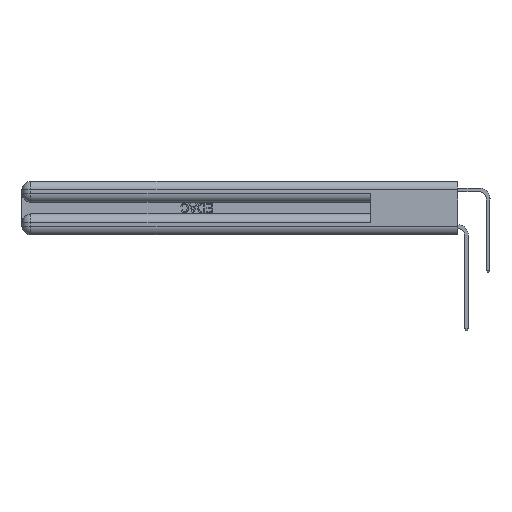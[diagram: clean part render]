
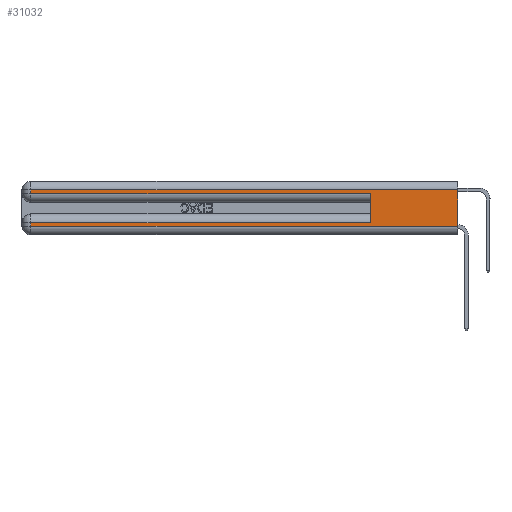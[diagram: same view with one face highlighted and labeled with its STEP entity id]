
A CAD part, left-side view. The second image highlights one B-rep face of the part: STEP entity #31032.
In plain terms, the highlighted planar face has unit normal (-1, 0, 0).
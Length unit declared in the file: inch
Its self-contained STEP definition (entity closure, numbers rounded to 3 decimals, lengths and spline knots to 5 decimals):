
#1410 = CARTESIAN_POINT ( 'NONE',  ( 0., 0.6, 0.285 ) ) ;
#1420 = ORIENTED_EDGE ( 'NONE', *, *, #5340, .F. ) ;
#1975 = LINE ( 'NONE', #37685, #36923 ) ;
#2135 = EDGE_CURVE ( 'NONE', #2789, #23034, #30403, .T. ) ;
#2245 = CARTESIAN_POINT ( 'NONE',  ( 0., 0., 0.285 ) ) ;
#2318 = EDGE_CURVE ( 'NONE', #9888, #27276, #2794, .T. ) ;
#2332 = VERTEX_POINT ( 'NONE', #26766 ) ;
#2610 = LINE ( 'NONE', #7416, #29763 ) ;
#2789 = VERTEX_POINT ( 'NONE', #29094 ) ;
#2794 = LINE ( 'NONE', #20740, #29479 ) ;
#3130 = CARTESIAN_POINT ( 'NONE',  ( 0., 2.94, 0.37 ) ) ;
#3451 = DIRECTION ( 'NONE',  ( 0., -1., 0. ) ) ;
#5340 = EDGE_CURVE ( 'NONE', #2789, #8459, #2610, .T. ) ;
#5794 = ORIENTED_EDGE ( 'NONE', *, *, #6654, .T. ) ;
#6057 = CARTESIAN_POINT ( 'NONE',  ( 0., 0., 0.06 ) ) ;
#6654 = EDGE_CURVE ( 'NONE', #16274, #27276, #7109, .T. ) ;
#6987 = CARTESIAN_POINT ( 'NONE',  ( 0., 0., 0.37 ) ) ;
#6991 = DIRECTION ( 'NONE',  ( 0., 1., 0. ) ) ;
#7109 = LINE ( 'NONE', #2245, #21837 ) ;
#7416 = CARTESIAN_POINT ( 'NONE',  ( 0., 0., 0.37 ) ) ;
#7418 = CARTESIAN_POINT ( 'NONE',  ( 0., 0.6, 0.085 ) ) ;
#8459 = VERTEX_POINT ( 'NONE', #6057 ) ;
#9888 = VERTEX_POINT ( 'NONE', #7418 ) ;
#10549 = VECTOR ( 'NONE', #19092, 39.37008 ) ;
#12088 = VECTOR ( 'NONE', #16734, 39.37008 ) ;
#12294 = DIRECTION ( 'NONE',  ( 0., 0., -1. ) ) ;
#13948 = LINE ( 'NONE', #14042, #12088 ) ;
#14042 = CARTESIAN_POINT ( 'NONE',  ( 0., 2.94, 0.37 ) ) ;
#15916 = DIRECTION ( 'NONE',  ( 0., 0., -1. ) ) ;
#15977 = EDGE_CURVE ( 'NONE', #9888, #2332, #22046, .T. ) ;
#16274 = VERTEX_POINT ( 'NONE', #29886 ) ;
#16606 = AXIS2_PLACEMENT_3D ( 'NONE', #6987, #29884, #12294 ) ;
#16734 = DIRECTION ( 'NONE',  ( 0., 0., -1. ) ) ;
#18335 = ORIENTED_EDGE ( 'NONE', *, *, #2135, .T. ) ;
#18462 = VECTOR ( 'NONE', #6991, 39.37008 ) ;
#19092 = DIRECTION ( 'NONE',  ( 0., 1., 0. ) ) ;
#20740 = CARTESIAN_POINT ( 'NONE',  ( 0., 0.6, 0.145 ) ) ;
#21837 = VECTOR ( 'NONE', #22852, 39.37008 ) ;
#22046 = LINE ( 'NONE', #36544, #10549 ) ;
#22135 = ORIENTED_EDGE ( 'NONE', *, *, #2318, .F. ) ;
#22368 = EDGE_CURVE ( 'NONE', #31572, #8459, #1975, .T. ) ;
#22852 = DIRECTION ( 'NONE',  ( 0., -1., 0. ) ) ;
#23034 = VERTEX_POINT ( 'NONE', #25589 ) ;
#23231 = DIRECTION ( 'NONE',  ( 0., 0., -1. ) ) ;
#23491 = CARTESIAN_POINT ( 'NONE',  ( 0., 0., 0.31 ) ) ;
#24449 = LINE ( 'NONE', #3130, #35050 ) ;
#24600 = PLANE ( 'NONE',  #16606 ) ;
#25589 = CARTESIAN_POINT ( 'NONE',  ( 0., 2.94, 0.31 ) ) ;
#26766 = CARTESIAN_POINT ( 'NONE',  ( 0., 2.94, 0.085 ) ) ;
#27276 = VERTEX_POINT ( 'NONE', #1410 ) ;
#29094 = CARTESIAN_POINT ( 'NONE',  ( 0., 0., 0.31 ) ) ;
#29373 = DIRECTION ( 'NONE',  ( 0., 0., 1. ) ) ;
#29479 = VECTOR ( 'NONE', #29373, 39.37008 ) ;
#29763 = VECTOR ( 'NONE', #15916, 39.37008 ) ;
#29884 = DIRECTION ( 'NONE',  ( 1., 0., 0. ) ) ;
#29886 = CARTESIAN_POINT ( 'NONE',  ( 0., 2.94, 0.285 ) ) ;
#30403 = LINE ( 'NONE', #23491, #18462 ) ;
#31032 = ADVANCED_FACE ( 'NONE', ( #32765 ), #24600, .F. ) ;
#31572 = VERTEX_POINT ( 'NONE', #33398 ) ;
#31779 = ORIENTED_EDGE ( 'NONE', *, *, #15977, .T. ) ;
#32765 = FACE_OUTER_BOUND ( 'NONE', #33131, .T. ) ;
#33131 = EDGE_LOOP ( 'NONE', ( #1420, #18335, #33409, #5794, #22135, #31779, #35691, #34311 ) ) ;
#33398 = CARTESIAN_POINT ( 'NONE',  ( 0., 2.94, 0.06 ) ) ;
#33409 = ORIENTED_EDGE ( 'NONE', *, *, #35151, .T. ) ;
#34311 = ORIENTED_EDGE ( 'NONE', *, *, #22368, .T. ) ;
#35050 = VECTOR ( 'NONE', #23231, 39.37008 ) ;
#35151 = EDGE_CURVE ( 'NONE', #23034, #16274, #13948, .T. ) ;
#35683 = EDGE_CURVE ( 'NONE', #2332, #31572, #24449, .T. ) ;
#35691 = ORIENTED_EDGE ( 'NONE', *, *, #35683, .T. ) ;
#36544 = CARTESIAN_POINT ( 'NONE',  ( 0., 0., 0.085 ) ) ;
#36923 = VECTOR ( 'NONE', #3451, 39.37008 ) ;
#37685 = CARTESIAN_POINT ( 'NONE',  ( 0., 0., 0.06 ) ) ;
